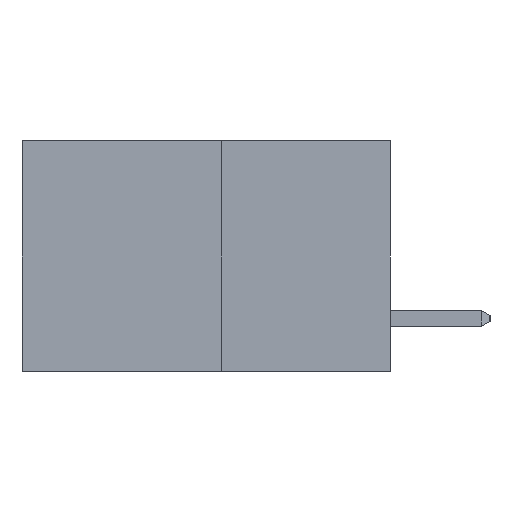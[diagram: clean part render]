
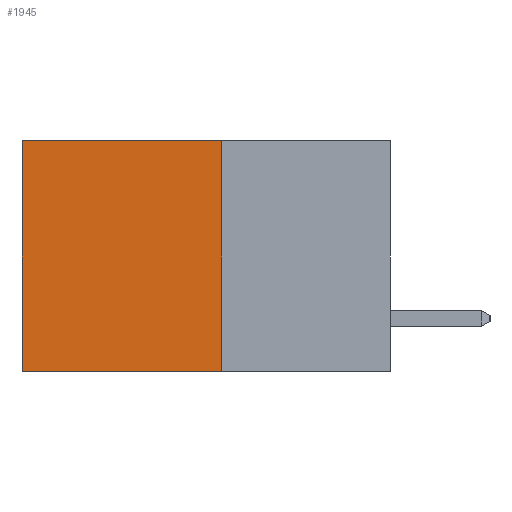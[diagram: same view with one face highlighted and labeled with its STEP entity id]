
A CAD part, left-side view. The second image highlights one B-rep face of the part: STEP entity #1945.
In plain terms, the highlighted planar face has unit normal (-1, 0, 0).
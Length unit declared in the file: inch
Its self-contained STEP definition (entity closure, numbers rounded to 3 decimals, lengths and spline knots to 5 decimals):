
#909 = VECTOR ( 'NONE', #10955, 39.37008 ) ;
#973 = EDGE_LOOP ( 'NONE', ( #13695, #12908, #10791, #12893 ) ) ;
#1243 = DIRECTION ( 'NONE',  ( 0., 0., -1. ) ) ;
#1945 = ADVANCED_FACE ( 'NONE', ( #4958 ), #11626, .F. ) ;
#2694 = CARTESIAN_POINT ( 'NONE',  ( 0.277, 0.59, -0.37 ) ) ;
#2802 = LINE ( 'NONE', #13489, #11753 ) ;
#4079 = VERTEX_POINT ( 'NONE', #6741 ) ;
#4771 = EDGE_CURVE ( 'NONE', #5549, #11715, #8134, .T. ) ;
#4778 = LINE ( 'NONE', #7216, #13649 ) ;
#4914 = EDGE_CURVE ( 'NONE', #4079, #5549, #2802, .T. ) ;
#4958 = FACE_OUTER_BOUND ( 'NONE', #973, .T. ) ;
#5549 = VERTEX_POINT ( 'NONE', #9074 ) ;
#6741 = CARTESIAN_POINT ( 'NONE',  ( 0.277, 0.27, 0. ) ) ;
#7216 = CARTESIAN_POINT ( 'NONE',  ( 0.277, 0.27, -0.37 ) ) ;
#7940 = EDGE_CURVE ( 'NONE', #12001, #11715, #13096, .T. ) ;
#8134 = LINE ( 'NONE', #14865, #11212 ) ;
#9074 = CARTESIAN_POINT ( 'NONE',  ( 0.277, 0.59, 0. ) ) ;
#9755 = AXIS2_PLACEMENT_3D ( 'NONE', #11808, #11748, #11729 ) ;
#10788 = CARTESIAN_POINT ( 'NONE',  ( 0.277, 0.27, -0.37 ) ) ;
#10791 = ORIENTED_EDGE ( 'NONE', *, *, #13698, .F. ) ;
#10955 = DIRECTION ( 'NONE',  ( 0., 1., 0. ) ) ;
#11212 = VECTOR ( 'NONE', #14796, 39.37008 ) ;
#11626 = PLANE ( 'NONE',  #9755 ) ;
#11660 = DIRECTION ( 'NONE',  ( 0., 1., 0. ) ) ;
#11715 = VERTEX_POINT ( 'NONE', #2694 ) ;
#11729 = DIRECTION ( 'NONE',  ( 0., 0., -1. ) ) ;
#11748 = DIRECTION ( 'NONE',  ( 1., 0., 0. ) ) ;
#11753 = VECTOR ( 'NONE', #11660, 39.37008 ) ;
#11808 = CARTESIAN_POINT ( 'NONE',  ( 0.277, 0.27, -0.37 ) ) ;
#12001 = VERTEX_POINT ( 'NONE', #14545 ) ;
#12893 = ORIENTED_EDGE ( 'NONE', *, *, #4914, .T. ) ;
#12908 = ORIENTED_EDGE ( 'NONE', *, *, #7940, .F. ) ;
#13096 = LINE ( 'NONE', #10788, #909 ) ;
#13489 = CARTESIAN_POINT ( 'NONE',  ( 0.277, 0.27, 0. ) ) ;
#13649 = VECTOR ( 'NONE', #1243, 39.37008 ) ;
#13695 = ORIENTED_EDGE ( 'NONE', *, *, #4771, .T. ) ;
#13698 = EDGE_CURVE ( 'NONE', #4079, #12001, #4778, .T. ) ;
#14545 = CARTESIAN_POINT ( 'NONE',  ( 0.277, 0.27, -0.37 ) ) ;
#14796 = DIRECTION ( 'NONE',  ( 0., 0., -1. ) ) ;
#14865 = CARTESIAN_POINT ( 'NONE',  ( 0.277, 0.59, -0.37 ) ) ;
